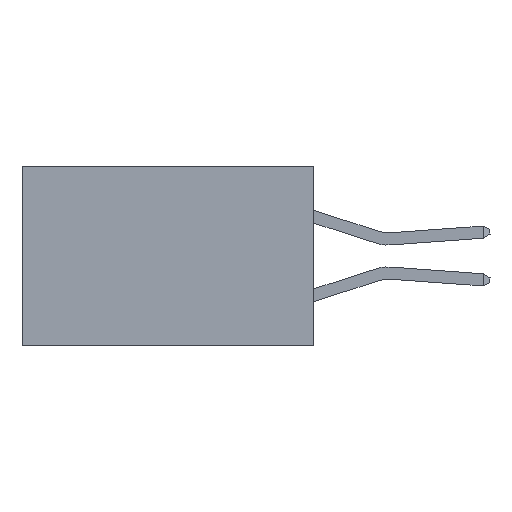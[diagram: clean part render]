
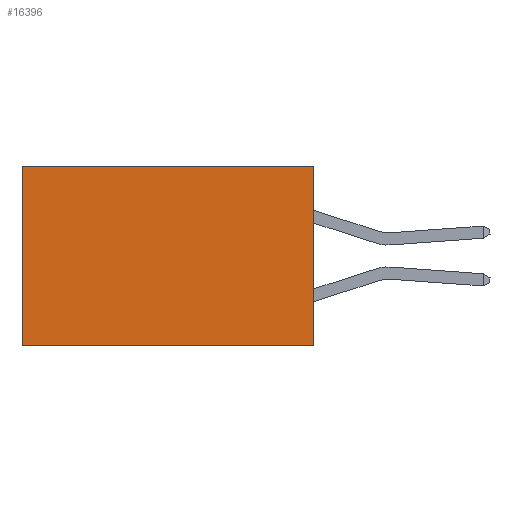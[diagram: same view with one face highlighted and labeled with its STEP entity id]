
A CAD part, left-side view. The second image highlights one B-rep face of the part: STEP entity #16396.
In plain terms, the highlighted planar face has unit normal (-1, 0, 0).
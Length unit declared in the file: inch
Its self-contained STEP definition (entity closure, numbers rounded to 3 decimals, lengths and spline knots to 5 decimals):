
#213 = EDGE_CURVE ( 'NONE', #22563, #36010, #9030, .T. ) ;
#700 = DIRECTION ( 'NONE',  ( 0., 0., -1. ) ) ;
#2733 = VERTEX_POINT ( 'NONE', #5442 ) ;
#2784 = DIRECTION ( 'NONE',  ( 0., 1., 0. ) ) ;
#3102 = PLANE ( 'NONE',  #30044 ) ;
#3269 = VECTOR ( 'NONE', #25458, 39.37008 ) ;
#4264 = LINE ( 'NONE', #16354, #3269 ) ;
#5442 = CARTESIAN_POINT ( 'NONE',  ( 0.2875, 0., -0.37 ) ) ;
#9030 = LINE ( 'NONE', #14885, #16341 ) ;
#11345 = VECTOR ( 'NONE', #700, 39.37008 ) ;
#14885 = CARTESIAN_POINT ( 'NONE',  ( 0.2875, 0.6, 0. ) ) ;
#14996 = ORIENTED_EDGE ( 'NONE', *, *, #16575, .F. ) ;
#15695 = DIRECTION ( 'NONE',  ( 1., 0., 0. ) ) ;
#16341 = VECTOR ( 'NONE', #28535, 39.37008 ) ;
#16354 = CARTESIAN_POINT ( 'NONE',  ( 0.2875, 0., -0.37 ) ) ;
#16396 = ADVANCED_FACE ( 'NONE', ( #32734 ), #3102, .F. ) ;
#16575 = EDGE_CURVE ( 'NONE', #2733, #36010, #4264, .T. ) ;
#19403 = CARTESIAN_POINT ( 'NONE',  ( 0.2875, 0., 0. ) ) ;
#20030 = EDGE_CURVE ( 'NONE', #21985, #22563, #20406, .T. ) ;
#20406 = LINE ( 'NONE', #24407, #35639 ) ;
#21985 = VERTEX_POINT ( 'NONE', #24361 ) ;
#22415 = ORIENTED_EDGE ( 'NONE', *, *, #213, .T. ) ;
#22563 = VERTEX_POINT ( 'NONE', #29879 ) ;
#23566 = EDGE_CURVE ( 'NONE', #21985, #2733, #38694, .T. ) ;
#24361 = CARTESIAN_POINT ( 'NONE',  ( 0.2875, 0., 0. ) ) ;
#24407 = CARTESIAN_POINT ( 'NONE',  ( 0.2875, 0., 0. ) ) ;
#25458 = DIRECTION ( 'NONE',  ( 0., 1., 0. ) ) ;
#26955 = ORIENTED_EDGE ( 'NONE', *, *, #23566, .F. ) ;
#27003 = CARTESIAN_POINT ( 'NONE',  ( 0.2875, 0., 0. ) ) ;
#28535 = DIRECTION ( 'NONE',  ( 0., 0., -1. ) ) ;
#29879 = CARTESIAN_POINT ( 'NONE',  ( 0.2875, 0.6, 0. ) ) ;
#30044 = AXIS2_PLACEMENT_3D ( 'NONE', #27003, #15695, #37033 ) ;
#30418 = EDGE_LOOP ( 'NONE', ( #22415, #14996, #26955, #32260 ) ) ;
#32260 = ORIENTED_EDGE ( 'NONE', *, *, #20030, .T. ) ;
#32644 = CARTESIAN_POINT ( 'NONE',  ( 0.2875, 0.6, -0.37 ) ) ;
#32734 = FACE_OUTER_BOUND ( 'NONE', #30418, .T. ) ;
#35639 = VECTOR ( 'NONE', #2784, 39.37008 ) ;
#36010 = VERTEX_POINT ( 'NONE', #32644 ) ;
#37033 = DIRECTION ( 'NONE',  ( 0., 0., -1. ) ) ;
#38694 = LINE ( 'NONE', #19403, #11345 ) ;
